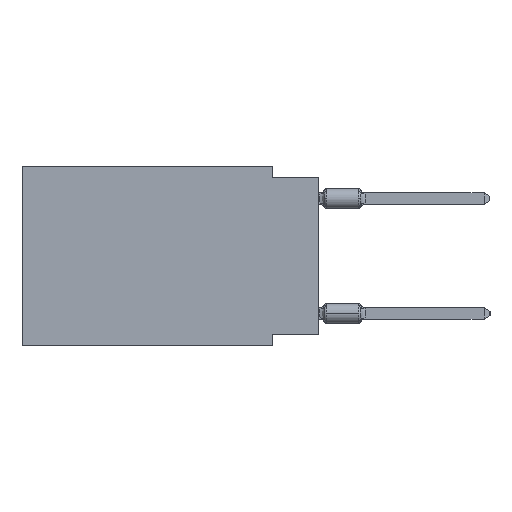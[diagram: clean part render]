
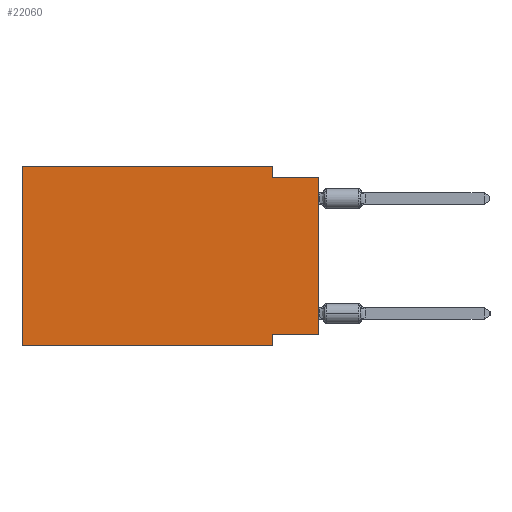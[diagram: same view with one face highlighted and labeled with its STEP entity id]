
A CAD part, left-side view. The second image highlights one B-rep face of the part: STEP entity #22060.
In plain terms, the highlighted planar face has unit normal (-1, 0, 0).
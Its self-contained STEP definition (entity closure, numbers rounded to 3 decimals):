
#1475 = EDGE_CURVE ( 'NONE', #21185, #33517, #47541, .T. ) ;
#1825 = VERTEX_POINT ( 'NONE', #9436 ) ;
#4795 = LINE ( 'NONE', #9590, #30674 ) ;
#6503 = CARTESIAN_POINT ( 'NONE',  ( 0., 16.383, 0. ) ) ;
#8841 = ORIENTED_EDGE ( 'NONE', *, *, #17329, .T. ) ;
#9420 = CARTESIAN_POINT ( 'NONE',  ( 0., 16.383, -9.906 ) ) ;
#9436 = CARTESIAN_POINT ( 'NONE',  ( 0., 2.54, -0.635 ) ) ;
#9590 = CARTESIAN_POINT ( 'NONE',  ( 0., 0., -0.635 ) ) ;
#10982 = EDGE_CURVE ( 'NONE', #13085, #30897, #13177, .T. ) ;
#11446 = ORIENTED_EDGE ( 'NONE', *, *, #44367, .F. ) ;
#13085 = VERTEX_POINT ( 'NONE', #41165 ) ;
#13177 = LINE ( 'NONE', #30547, #41735 ) ;
#14287 = EDGE_CURVE ( 'NONE', #33517, #39404, #22755, .T. ) ;
#14581 = LINE ( 'NONE', #24474, #46923 ) ;
#15717 = CARTESIAN_POINT ( 'NONE',  ( 0., 16.383, 0. ) ) ;
#17329 = EDGE_CURVE ( 'NONE', #13085, #53242, #14581, .T. ) ;
#17488 = CARTESIAN_POINT ( 'NONE',  ( 0., 2.54, 0. ) ) ;
#18529 = CARTESIAN_POINT ( 'NONE',  ( 0., 2.54, -9.906 ) ) ;
#19160 = CARTESIAN_POINT ( 'NONE',  ( 0., 2.54, -9.271 ) ) ;
#20368 = EDGE_CURVE ( 'NONE', #30897, #45630, #48316, .T. ) ;
#21076 = PLANE ( 'NONE',  #37488 ) ;
#21185 = VERTEX_POINT ( 'NONE', #44491 ) ;
#21274 = DIRECTION ( 'NONE',  ( 0., 0., -1. ) ) ;
#22060 = ADVANCED_FACE ( 'NONE', ( #38748 ), #21076, .F. ) ;
#22474 = DIRECTION ( 'NONE',  ( 0., 0., -1. ) ) ;
#22755 = LINE ( 'NONE', #23036, #26573 ) ;
#23036 = CARTESIAN_POINT ( 'NONE',  ( 0., 16.383, 0. ) ) ;
#23357 = VECTOR ( 'NONE', #21274, 1000. ) ;
#24169 = DIRECTION ( 'NONE',  ( 0., 0., 1. ) ) ;
#24474 = CARTESIAN_POINT ( 'NONE',  ( 0., 0., 0. ) ) ;
#24835 = ORIENTED_EDGE ( 'NONE', *, *, #10982, .F. ) ;
#25159 = EDGE_LOOP ( 'NONE', ( #8841, #27895, #11446, #37928, #41602, #44971, #55297, #24835 ) ) ;
#26573 = VECTOR ( 'NONE', #49413, 1000. ) ;
#27895 = ORIENTED_EDGE ( 'NONE', *, *, #32511, .F. ) ;
#30547 = CARTESIAN_POINT ( 'NONE',  ( 0., 0., -9.271 ) ) ;
#30674 = VECTOR ( 'NONE', #51230, 1000. ) ;
#30897 = VERTEX_POINT ( 'NONE', #19160 ) ;
#31968 = CARTESIAN_POINT ( 'NONE',  ( 0., 16.383, 0. ) ) ;
#32511 = EDGE_CURVE ( 'NONE', #1825, #53242, #4795, .T. ) ;
#32852 = DIRECTION ( 'NONE',  ( 0., 0., 1. ) ) ;
#33517 = VERTEX_POINT ( 'NONE', #31968 ) ;
#37488 = AXIS2_PLACEMENT_3D ( 'NONE', #15717, #44428, #44121 ) ;
#37536 = DIRECTION ( 'NONE',  ( 0., -1., 0. ) ) ;
#37928 = ORIENTED_EDGE ( 'NONE', *, *, #14287, .F. ) ;
#38748 = FACE_OUTER_BOUND ( 'NONE', #25159, .T. ) ;
#39404 = VERTEX_POINT ( 'NONE', #17488 ) ;
#41165 = CARTESIAN_POINT ( 'NONE',  ( 0., 0., -9.271 ) ) ;
#41602 = ORIENTED_EDGE ( 'NONE', *, *, #1475, .F. ) ;
#41735 = VECTOR ( 'NONE', #48829, 1000. ) ;
#44103 = CARTESIAN_POINT ( 'NONE',  ( 0., 2.54, -9.906 ) ) ;
#44121 = DIRECTION ( 'NONE',  ( 0., 0., -1. ) ) ;
#44331 = LINE ( 'NONE', #52730, #23357 ) ;
#44367 = EDGE_CURVE ( 'NONE', #39404, #1825, #44331, .T. ) ;
#44428 = DIRECTION ( 'NONE',  ( 1., 0., 0. ) ) ;
#44491 = CARTESIAN_POINT ( 'NONE',  ( 0., 16.383, -9.906 ) ) ;
#44869 = VECTOR ( 'NONE', #37536, 1000. ) ;
#44971 = ORIENTED_EDGE ( 'NONE', *, *, #54444, .T. ) ;
#45630 = VERTEX_POINT ( 'NONE', #18529 ) ;
#46053 = VECTOR ( 'NONE', #22474, 1000. ) ;
#46246 = LINE ( 'NONE', #9420, #44869 ) ;
#46923 = VECTOR ( 'NONE', #24169, 1000. ) ;
#47085 = VECTOR ( 'NONE', #32852, 1000. ) ;
#47541 = LINE ( 'NONE', #6503, #47085 ) ;
#48316 = LINE ( 'NONE', #44103, #46053 ) ;
#48829 = DIRECTION ( 'NONE',  ( 0., 1., 0. ) ) ;
#49413 = DIRECTION ( 'NONE',  ( 0., -1., 0. ) ) ;
#51230 = DIRECTION ( 'NONE',  ( 0., -1., 0. ) ) ;
#52730 = CARTESIAN_POINT ( 'NONE',  ( 0., 2.54, 0. ) ) ;
#53242 = VERTEX_POINT ( 'NONE', #57775 ) ;
#54444 = EDGE_CURVE ( 'NONE', #21185, #45630, #46246, .T. ) ;
#55297 = ORIENTED_EDGE ( 'NONE', *, *, #20368, .F. ) ;
#57775 = CARTESIAN_POINT ( 'NONE',  ( 0., 0., -0.635 ) ) ;
